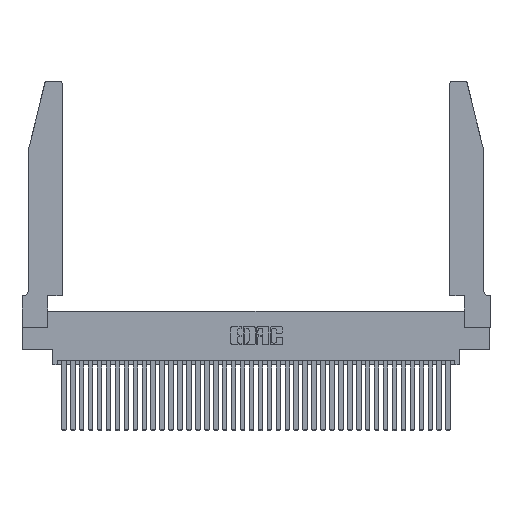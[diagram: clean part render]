
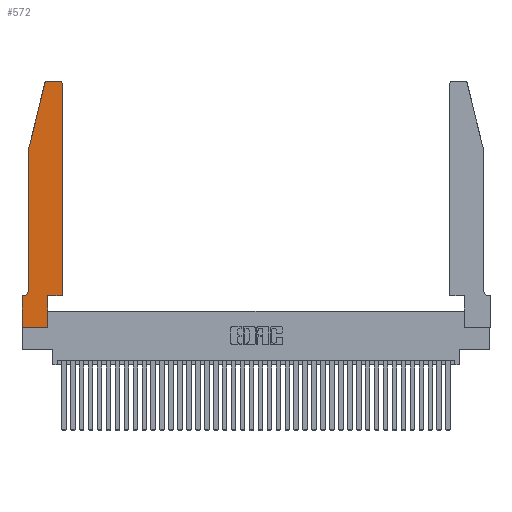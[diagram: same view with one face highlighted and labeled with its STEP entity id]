
A CAD part, top view. The second image highlights one B-rep face of the part: STEP entity #572.
In plain terms, the highlighted planar face has unit normal (0, 0, 1).
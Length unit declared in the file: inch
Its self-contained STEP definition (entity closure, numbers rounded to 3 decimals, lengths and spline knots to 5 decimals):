
#257 = LINE ( 'NONE', #29750, #21393 ) ;
#371 = VECTOR ( 'NONE', #26951, 39.37008 ) ;
#572 = ADVANCED_FACE ( 'NONE', ( #10818 ), #20552, .T. ) ;
#918 = ORIENTED_EDGE ( 'NONE', *, *, #6437, .T. ) ;
#2803 = VERTEX_POINT ( 'NONE', #19853 ) ;
#4177 = AXIS2_PLACEMENT_3D ( 'NONE', #17561, #38661, #20602 ) ;
#4268 = VECTOR ( 'NONE', #5344, 39.37008 ) ;
#4288 = VERTEX_POINT ( 'NONE', #23184 ) ;
#4354 = ORIENTED_EDGE ( 'NONE', *, *, #33449, .T. ) ;
#4694 = VERTEX_POINT ( 'NONE', #5178 ) ;
#5178 = CARTESIAN_POINT ( 'NONE',  ( 0., 0.35, 0.37 ) ) ;
#5344 = DIRECTION ( 'NONE',  ( -0.239, -0.971, 0. ) ) ;
#5411 = LINE ( 'NONE', #18829, #14363 ) ;
#5803 = CARTESIAN_POINT ( 'NONE',  ( 0.0755, 0.35, 0.37 ) ) ;
#6437 = EDGE_CURVE ( 'NONE', #30953, #2803, #25424, .T. ) ;
#6603 = CARTESIAN_POINT ( 'NONE',  ( 0.2865, 0., 0.37 ) ) ;
#7074 = VECTOR ( 'NONE', #29623, 39.37008 ) ;
#7411 = AXIS2_PLACEMENT_3D ( 'NONE', #23609, #29647, #11670 ) ;
#7771 = EDGE_CURVE ( 'NONE', #4694, #20589, #31407, .T. ) ;
#8139 = CARTESIAN_POINT ( 'NONE',  ( 0.284, 2.72, 0.37 ) ) ;
#8229 = AXIS2_PLACEMENT_3D ( 'NONE', #8139, #17280, #11702 ) ;
#8735 = DIRECTION ( 'NONE',  ( -1., 0., 0. ) ) ;
#8934 = DIRECTION ( 'NONE',  ( 1., 0., 0. ) ) ;
#9068 = CARTESIAN_POINT ( 'NONE',  ( 0.25487, 2.72718, 0.37 ) ) ;
#9612 = CIRCLE ( 'NONE', #8229, 0.03 ) ;
#9753 = VERTEX_POINT ( 'NONE', #26485 ) ;
#9993 = EDGE_CURVE ( 'NONE', #21391, #4288, #5411, .T. ) ;
#10818 = FACE_OUTER_BOUND ( 'NONE', #25749, .T. ) ;
#11670 = DIRECTION ( 'NONE',  ( 1., 0., 0. ) ) ;
#11702 = DIRECTION ( 'NONE',  ( 1., 0., 0. ) ) ;
#11793 = ORIENTED_EDGE ( 'NONE', *, *, #27490, .T. ) ;
#13040 = ORIENTED_EDGE ( 'NONE', *, *, #34466, .T. ) ;
#14357 = DIRECTION ( 'NONE',  ( 1., 0., 0. ) ) ;
#14363 = VECTOR ( 'NONE', #34518, 39.37008 ) ;
#14654 = LINE ( 'NONE', #5803, #26908 ) ;
#15230 = EDGE_CURVE ( 'NONE', #4288, #38216, #22020, .T. ) ;
#15399 = ORIENTED_EDGE ( 'NONE', *, *, #9993, .T. ) ;
#15428 = ORIENTED_EDGE ( 'NONE', *, *, #15230, .T. ) ;
#15628 = VECTOR ( 'NONE', #8934, 39.37008 ) ;
#15939 = CARTESIAN_POINT ( 'NONE',  ( 0.0055, 0.42, 0.37 ) ) ;
#16809 = CARTESIAN_POINT ( 'NONE',  ( 0.2865, 0.35, 0.37 ) ) ;
#17280 = DIRECTION ( 'NONE',  ( 0., 0., 1. ) ) ;
#17561 = CARTESIAN_POINT ( 'NONE',  ( 0.4205, 2.72, 0.37 ) ) ;
#17596 = CARTESIAN_POINT ( 'NONE',  ( 0.2605, 2.75, 0.37 ) ) ;
#17927 = VERTEX_POINT ( 'NONE', #6603 ) ;
#18408 = VERTEX_POINT ( 'NONE', #35262 ) ;
#18509 = VERTEX_POINT ( 'NONE', #16809 ) ;
#18829 = CARTESIAN_POINT ( 'NONE',  ( 0.4505, 0.35, 0.37 ) ) ;
#19084 = CARTESIAN_POINT ( 'NONE',  ( 0.0755, 2., 0.37 ) ) ;
#19853 = CARTESIAN_POINT ( 'NONE',  ( 0.0755, 0.42, 0.37 ) ) ;
#19983 = DIRECTION ( 'NONE',  ( 0., -1., 0. ) ) ;
#20322 = LINE ( 'NONE', #22945, #15628 ) ;
#20528 = CARTESIAN_POINT ( 'NONE',  ( 0.0755, 2., 0.37 ) ) ;
#20552 = PLANE ( 'NONE',  #7411 ) ;
#20568 = LINE ( 'NONE', #36153, #371 ) ;
#20589 = VERTEX_POINT ( 'NONE', #38949 ) ;
#20602 = DIRECTION ( 'NONE',  ( 1., 0., 0. ) ) ;
#21155 = EDGE_CURVE ( 'NONE', #9753, #27588, #9612, .T. ) ;
#21391 = VERTEX_POINT ( 'NONE', #21861 ) ;
#21393 = VECTOR ( 'NONE', #14357, 39.37008 ) ;
#21861 = CARTESIAN_POINT ( 'NONE',  ( 0.4505, 0.35, 0.37 ) ) ;
#22020 = CIRCLE ( 'NONE', #4177, 0.03 ) ;
#22314 = EDGE_CURVE ( 'NONE', #38216, #9753, #28771, .T. ) ;
#22945 = CARTESIAN_POINT ( 'NONE',  ( 0.4505, 0.35, 0.37 ) ) ;
#23184 = CARTESIAN_POINT ( 'NONE',  ( 0.4505, 2.72, 0.37 ) ) ;
#23352 = ORIENTED_EDGE ( 'NONE', *, *, #21155, .T. ) ;
#23424 = DIRECTION ( 'NONE',  ( -1., 0., 0. ) ) ;
#23609 = CARTESIAN_POINT ( 'NONE',  ( 0., 0.35, 0.37 ) ) ;
#23937 = VECTOR ( 'NONE', #19983, 39.37008 ) ;
#23984 = ORIENTED_EDGE ( 'NONE', *, *, #22314, .T. ) ;
#24378 = AXIS2_PLACEMENT_3D ( 'NONE', #15939, #30957, #24673 ) ;
#24469 = CIRCLE ( 'NONE', #24378, 0.07 ) ;
#24673 = DIRECTION ( 'NONE',  ( -1., 0., 0. ) ) ;
#25275 = CARTESIAN_POINT ( 'NONE',  ( 0.4205, 2.75, 0.37 ) ) ;
#25424 = LINE ( 'NONE', #20528, #7074 ) ;
#25449 = LINE ( 'NONE', #34982, #4268 ) ;
#25749 = EDGE_LOOP ( 'NONE', ( #23984, #23352, #27066, #918, #4354, #38034, #27443, #29882, #13040, #11793, #15399, #15428 ) ) ;
#26485 = CARTESIAN_POINT ( 'NONE',  ( 0.284, 2.75, 0.37 ) ) ;
#26908 = VECTOR ( 'NONE', #8735, 39.37008 ) ;
#26951 = DIRECTION ( 'NONE',  ( 0., 1., 0. ) ) ;
#27066 = ORIENTED_EDGE ( 'NONE', *, *, #28665, .T. ) ;
#27443 = ORIENTED_EDGE ( 'NONE', *, *, #7771, .T. ) ;
#27490 = EDGE_CURVE ( 'NONE', #18509, #21391, #20322, .T. ) ;
#27588 = VERTEX_POINT ( 'NONE', #9068 ) ;
#28205 = EDGE_CURVE ( 'NONE', #18408, #4694, #14654, .T. ) ;
#28309 = CARTESIAN_POINT ( 'NONE',  ( 0., 0., 0.37 ) ) ;
#28665 = EDGE_CURVE ( 'NONE', #27588, #30953, #25449, .T. ) ;
#28771 = LINE ( 'NONE', #17596, #38206 ) ;
#29623 = DIRECTION ( 'NONE',  ( 0., -1., 0. ) ) ;
#29647 = DIRECTION ( 'NONE',  ( 0., 0., 1. ) ) ;
#29750 = CARTESIAN_POINT ( 'NONE',  ( 0., 0., 0.37 ) ) ;
#29882 = ORIENTED_EDGE ( 'NONE', *, *, #35595, .T. ) ;
#30953 = VERTEX_POINT ( 'NONE', #19084 ) ;
#30957 = DIRECTION ( 'NONE',  ( 0., 0., -1. ) ) ;
#31407 = LINE ( 'NONE', #28309, #23937 ) ;
#33449 = EDGE_CURVE ( 'NONE', #2803, #18408, #24469, .T. ) ;
#34466 = EDGE_CURVE ( 'NONE', #17927, #18509, #20568, .T. ) ;
#34518 = DIRECTION ( 'NONE',  ( 0., 1., 0. ) ) ;
#34982 = CARTESIAN_POINT ( 'NONE',  ( 0.0755, 2., 0.37 ) ) ;
#35262 = CARTESIAN_POINT ( 'NONE',  ( 0.0055, 0.35, 0.37 ) ) ;
#35595 = EDGE_CURVE ( 'NONE', #20589, #17927, #257, .T. ) ;
#36153 = CARTESIAN_POINT ( 'NONE',  ( 0.2865, 0.35, 0.37 ) ) ;
#38034 = ORIENTED_EDGE ( 'NONE', *, *, #28205, .T. ) ;
#38206 = VECTOR ( 'NONE', #23424, 39.37008 ) ;
#38216 = VERTEX_POINT ( 'NONE', #25275 ) ;
#38661 = DIRECTION ( 'NONE',  ( 0., 0., 1. ) ) ;
#38949 = CARTESIAN_POINT ( 'NONE',  ( 0., 0., 0.37 ) ) ;
